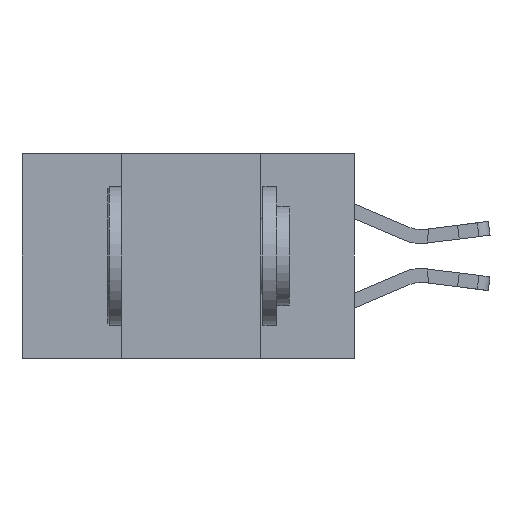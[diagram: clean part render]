
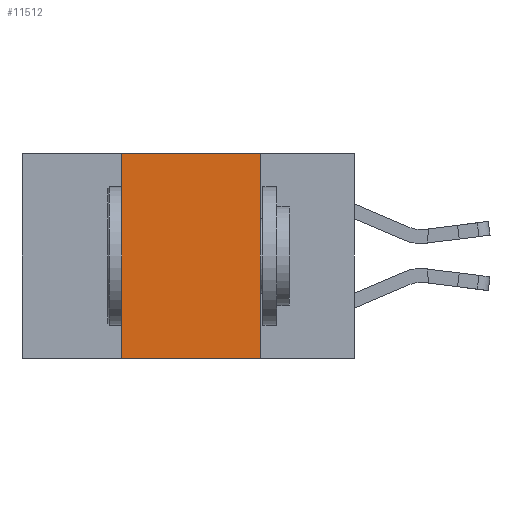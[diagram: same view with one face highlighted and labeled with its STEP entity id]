
A CAD part, left-side view. The second image highlights one B-rep face of the part: STEP entity #11512.
In plain terms, the highlighted planar face has unit normal (-1, 0, 0).
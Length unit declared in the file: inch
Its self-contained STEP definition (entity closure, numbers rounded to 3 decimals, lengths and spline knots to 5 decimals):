
#321 = VERTEX_POINT ( 'NONE', #11935 ) ;
#877 = DIRECTION ( 'NONE',  ( 1., 0., 0. ) ) ;
#2138 = FACE_OUTER_BOUND ( 'NONE', #8202, .T. ) ;
#3217 = LINE ( 'NONE', #11455, #8561 ) ;
#3752 = DIRECTION ( 'NONE',  ( 0., -1., 0. ) ) ;
#4753 = VERTEX_POINT ( 'NONE', #12240 ) ;
#4878 = DIRECTION ( 'NONE',  ( 0., 0., 1. ) ) ;
#5766 = VECTOR ( 'NONE', #6038, 39.37008 ) ;
#5859 = LINE ( 'NONE', #10852, #14551 ) ;
#5975 = EDGE_CURVE ( 'NONE', #4753, #10345, #5859, .T. ) ;
#6015 = CARTESIAN_POINT ( 'NONE',  ( 0., 0.6, 0. ) ) ;
#6038 = DIRECTION ( 'NONE',  ( 0., -1., 0. ) ) ;
#6769 = EDGE_CURVE ( 'NONE', #4753, #13887, #9235, .T. ) ;
#6952 = ORIENTED_EDGE ( 'NONE', *, *, #10010, .F. ) ;
#7726 = ORIENTED_EDGE ( 'NONE', *, *, #6769, .F. ) ;
#7988 = CARTESIAN_POINT ( 'NONE',  ( 0., 0.42, 0. ) ) ;
#8083 = ORIENTED_EDGE ( 'NONE', *, *, #5975, .T. ) ;
#8202 = EDGE_LOOP ( 'NONE', ( #6952, #13243, #7726, #8083 ) ) ;
#8561 = VECTOR ( 'NONE', #9151, 39.37008 ) ;
#8731 = EDGE_CURVE ( 'NONE', #13887, #321, #14804, .T. ) ;
#9151 = DIRECTION ( 'NONE',  ( 0., 0., -1. ) ) ;
#9235 = LINE ( 'NONE', #7988, #14686 ) ;
#9519 = DIRECTION ( 'NONE',  ( 0., 0., -1. ) ) ;
#9762 = CARTESIAN_POINT ( 'NONE',  ( 0., 0.17, -0.37 ) ) ;
#10010 = EDGE_CURVE ( 'NONE', #321, #10345, #3217, .T. ) ;
#10345 = VERTEX_POINT ( 'NONE', #9762 ) ;
#10805 = AXIS2_PLACEMENT_3D ( 'NONE', #14135, #877, #9519 ) ;
#10852 = CARTESIAN_POINT ( 'NONE',  ( 0., 0.6, -0.37 ) ) ;
#11455 = CARTESIAN_POINT ( 'NONE',  ( 0., 0.17, 0. ) ) ;
#11512 = ADVANCED_FACE ( 'NONE', ( #2138 ), #15279, .F. ) ;
#11935 = CARTESIAN_POINT ( 'NONE',  ( 0., 0.17, 0. ) ) ;
#12240 = CARTESIAN_POINT ( 'NONE',  ( 0., 0.42, -0.37 ) ) ;
#13243 = ORIENTED_EDGE ( 'NONE', *, *, #8731, .F. ) ;
#13887 = VERTEX_POINT ( 'NONE', #15380 ) ;
#14135 = CARTESIAN_POINT ( 'NONE',  ( 0., 0.6, 0. ) ) ;
#14551 = VECTOR ( 'NONE', #3752, 39.37008 ) ;
#14686 = VECTOR ( 'NONE', #4878, 39.37008 ) ;
#14804 = LINE ( 'NONE', #6015, #5766 ) ;
#15279 = PLANE ( 'NONE',  #10805 ) ;
#15380 = CARTESIAN_POINT ( 'NONE',  ( 0., 0.42, 0. ) ) ;
